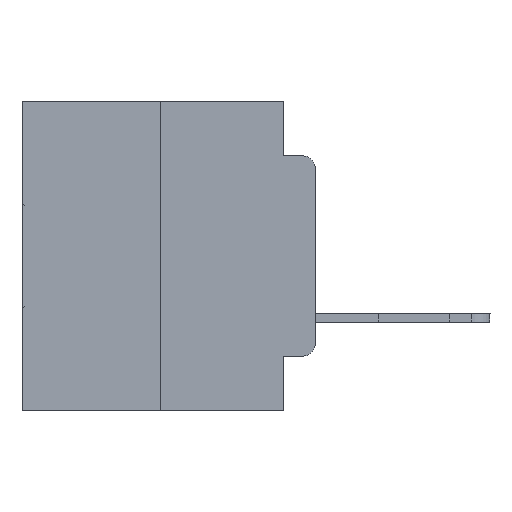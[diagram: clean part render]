
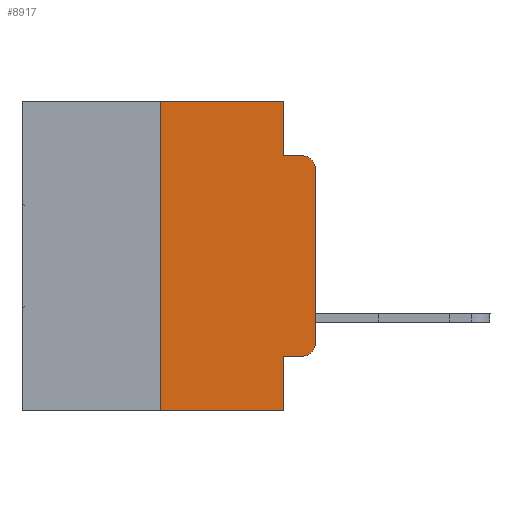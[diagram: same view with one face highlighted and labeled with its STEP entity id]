
A CAD part, left-side view. The second image highlights one B-rep face of the part: STEP entity #8917.
In plain terms, the highlighted planar face has unit normal (-1, 0, 0).
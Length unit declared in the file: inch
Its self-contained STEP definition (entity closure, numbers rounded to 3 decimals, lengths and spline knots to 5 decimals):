
#811 = EDGE_CURVE ( 'NONE', #3876, #4799, #8134, .T. ) ;
#1395 = DIRECTION ( 'NONE',  ( 0., -1., 0. ) ) ;
#1627 = CARTESIAN_POINT ( 'NONE',  ( 0., 0.473, 0. ) ) ;
#1647 = CARTESIAN_POINT ( 'NONE',  ( 0., 0., -0.3915 ) ) ;
#2135 = LINE ( 'NONE', #15864, #11272 ) ;
#2162 = ORIENTED_EDGE ( 'NONE', *, *, #29460, .F. ) ;
#2500 = CARTESIAN_POINT ( 'NONE',  ( 0., 0.25, 0. ) ) ;
#2839 = CARTESIAN_POINT ( 'NONE',  ( 0., 0., 0. ) ) ;
#3127 = LINE ( 'NONE', #14735, #22619 ) ;
#3552 = CARTESIAN_POINT ( 'NONE',  ( 0., 0.051, -0.5 ) ) ;
#3844 = ORIENTED_EDGE ( 'NONE', *, *, #23709, .T. ) ;
#3876 = VERTEX_POINT ( 'NONE', #2500 ) ;
#4328 = LINE ( 'NONE', #8385, #19612 ) ;
#4376 = VERTEX_POINT ( 'NONE', #27792 ) ;
#4799 = VERTEX_POINT ( 'NONE', #16736 ) ;
#5244 = AXIS2_PLACEMENT_3D ( 'NONE', #18878, #14343, #21441 ) ;
#5549 = EDGE_LOOP ( 'NONE', ( #15229, #3844, #16788, #2162, #13015, #23343, #8924, #13617, #14420, #21190 ) ) ;
#5852 = DIRECTION ( 'NONE',  ( 0., 0., -1. ) ) ;
#8134 = LINE ( 'NONE', #17352, #10697 ) ;
#8385 = CARTESIAN_POINT ( 'NONE',  ( 0., 0.051, -0.4115 ) ) ;
#8413 = FACE_OUTER_BOUND ( 'NONE', #5549, .T. ) ;
#8535 = DIRECTION ( 'NONE',  ( 0., 0., -1. ) ) ;
#8762 = DIRECTION ( 'NONE',  ( 0., 0., 1. ) ) ;
#8914 = VECTOR ( 'NONE', #1395, 39.37008 ) ;
#8917 = ADVANCED_FACE ( 'NONE', ( #8413 ), #17793, .F. ) ;
#8924 = ORIENTED_EDGE ( 'NONE', *, *, #21549, .T. ) ;
#8989 = EDGE_CURVE ( 'NONE', #18078, #22108, #3127, .T. ) ;
#9897 = EDGE_CURVE ( 'NONE', #22676, #18946, #10989, .T. ) ;
#10278 = LINE ( 'NONE', #21630, #21115 ) ;
#10628 = DIRECTION ( 'NONE',  ( -1., 0., 0. ) ) ;
#10697 = VECTOR ( 'NONE', #22033, 39.37008 ) ;
#10989 = CIRCLE ( 'NONE', #5244, 0.02 ) ;
#11078 = CARTESIAN_POINT ( 'NONE',  ( 0., 0.02, -0.1085 ) ) ;
#11272 = VECTOR ( 'NONE', #8762, 39.37008 ) ;
#12322 = DIRECTION ( 'NONE',  ( 0., 0., -1. ) ) ;
#13015 = ORIENTED_EDGE ( 'NONE', *, *, #811, .F. ) ;
#13617 = ORIENTED_EDGE ( 'NONE', *, *, #8989, .F. ) ;
#13731 = VECTOR ( 'NONE', #27748, 39.37008 ) ;
#14343 = DIRECTION ( 'NONE',  ( -1., 0., 0. ) ) ;
#14420 = ORIENTED_EDGE ( 'NONE', *, *, #24954, .T. ) ;
#14464 = CARTESIAN_POINT ( 'NONE',  ( 0., 0.051, 0. ) ) ;
#14520 = CARTESIAN_POINT ( 'NONE',  ( 0., 0.02, -0.0885 ) ) ;
#14735 = CARTESIAN_POINT ( 'NONE',  ( 0., 0.051, 0. ) ) ;
#15179 = DIRECTION ( 'NONE',  ( 0., -1., 0. ) ) ;
#15229 = ORIENTED_EDGE ( 'NONE', *, *, #17111, .T. ) ;
#15864 = CARTESIAN_POINT ( 'NONE',  ( 0., 0.25, 0. ) ) ;
#16733 = LINE ( 'NONE', #14464, #13731 ) ;
#16736 = CARTESIAN_POINT ( 'NONE',  ( 0., 0.051, 0. ) ) ;
#16788 = ORIENTED_EDGE ( 'NONE', *, *, #25687, .F. ) ;
#17111 = EDGE_CURVE ( 'NONE', #18946, #17646, #21113, .T. ) ;
#17352 = CARTESIAN_POINT ( 'NONE',  ( 0., 0.473, 0. ) ) ;
#17646 = VERTEX_POINT ( 'NONE', #21941 ) ;
#17793 = PLANE ( 'NONE',  #25478 ) ;
#18078 = VERTEX_POINT ( 'NONE', #25268 ) ;
#18203 = CIRCLE ( 'NONE', #29760, 0.02 ) ;
#18878 = CARTESIAN_POINT ( 'NONE',  ( 0., 0.02, -0.3915 ) ) ;
#18917 = CARTESIAN_POINT ( 'NONE',  ( 0., 0.25, -0.5 ) ) ;
#18946 = VERTEX_POINT ( 'NONE', #1647 ) ;
#19612 = VECTOR ( 'NONE', #15179, 39.37008 ) ;
#21113 = LINE ( 'NONE', #2839, #25160 ) ;
#21115 = VECTOR ( 'NONE', #23615, 39.37008 ) ;
#21190 = ORIENTED_EDGE ( 'NONE', *, *, #9897, .T. ) ;
#21441 = DIRECTION ( 'NONE',  ( 0., 0., -1. ) ) ;
#21549 = EDGE_CURVE ( 'NONE', #27400, #22108, #24338, .T. ) ;
#21630 = CARTESIAN_POINT ( 'NONE',  ( 0., 0.051, -0.0885 ) ) ;
#21941 = CARTESIAN_POINT ( 'NONE',  ( 0., 0., -0.1085 ) ) ;
#22033 = DIRECTION ( 'NONE',  ( 0., -1., 0. ) ) ;
#22108 = VERTEX_POINT ( 'NONE', #3552 ) ;
#22619 = VECTOR ( 'NONE', #12322, 39.37008 ) ;
#22676 = VERTEX_POINT ( 'NONE', #26024 ) ;
#23232 = DIRECTION ( 'NONE',  ( 0., 0., 1. ) ) ;
#23343 = ORIENTED_EDGE ( 'NONE', *, *, #28821, .F. ) ;
#23615 = DIRECTION ( 'NONE',  ( 0., -1., 0. ) ) ;
#23709 = EDGE_CURVE ( 'NONE', #17646, #27362, #18203, .T. ) ;
#24338 = LINE ( 'NONE', #28998, #8914 ) ;
#24954 = EDGE_CURVE ( 'NONE', #18078, #22676, #4328, .T. ) ;
#25160 = VECTOR ( 'NONE', #23232, 39.37008 ) ;
#25268 = CARTESIAN_POINT ( 'NONE',  ( 0., 0.051, -0.4115 ) ) ;
#25478 = AXIS2_PLACEMENT_3D ( 'NONE', #1627, #26520, #5852 ) ;
#25687 = EDGE_CURVE ( 'NONE', #4376, #27362, #10278, .T. ) ;
#26024 = CARTESIAN_POINT ( 'NONE',  ( 0., 0.02, -0.4115 ) ) ;
#26520 = DIRECTION ( 'NONE',  ( 1., 0., 0. ) ) ;
#27362 = VERTEX_POINT ( 'NONE', #14520 ) ;
#27400 = VERTEX_POINT ( 'NONE', #18917 ) ;
#27748 = DIRECTION ( 'NONE',  ( 0., 0., -1. ) ) ;
#27792 = CARTESIAN_POINT ( 'NONE',  ( 0., 0.051, -0.0885 ) ) ;
#28821 = EDGE_CURVE ( 'NONE', #27400, #3876, #2135, .T. ) ;
#28998 = CARTESIAN_POINT ( 'NONE',  ( 0., 0.473, -0.5 ) ) ;
#29460 = EDGE_CURVE ( 'NONE', #4799, #4376, #16733, .T. ) ;
#29760 = AXIS2_PLACEMENT_3D ( 'NONE', #11078, #10628, #8535 ) ;
